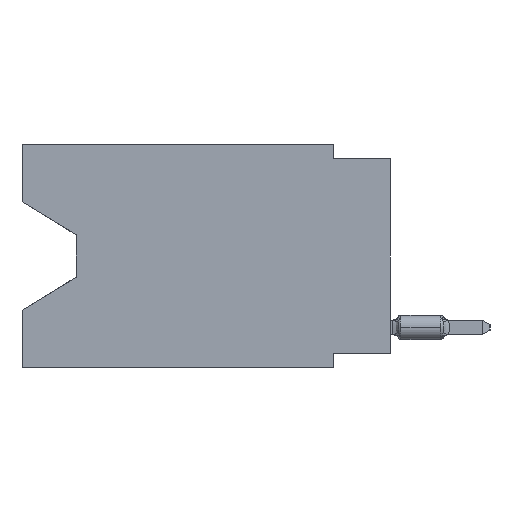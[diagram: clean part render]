
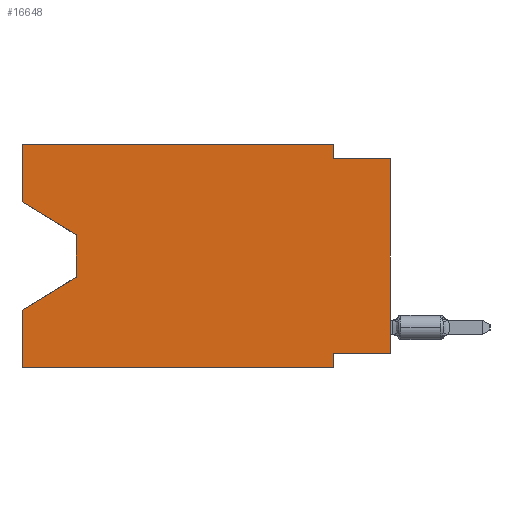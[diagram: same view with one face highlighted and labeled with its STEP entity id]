
A CAD part, left-side view. The second image highlights one B-rep face of the part: STEP entity #16648.
In plain terms, the highlighted planar face has unit normal (-1, 0, 0).
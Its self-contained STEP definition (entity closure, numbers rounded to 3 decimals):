
#16 = ORIENTED_EDGE ( 'NONE', *, *, #13307, .T. ) ;
#127 = EDGE_CURVE ( 'NONE', #4438, #49272, #79019, .T. ) ;
#498 = VERTEX_POINT ( 'NONE', #81264 ) ;
#1169 = CARTESIAN_POINT ( 'NONE',  ( 0., 0., 0. ) ) ;
#1260 = CARTESIAN_POINT ( 'NONE',  ( 0., 2.54, -0.635 ) ) ;
#3491 = ORIENTED_EDGE ( 'NONE', *, *, #4138, .F. ) ;
#4138 = EDGE_CURVE ( 'NONE', #498, #16381, #55338, .T. ) ;
#4438 = VERTEX_POINT ( 'NONE', #1260 ) ;
#4476 = DIRECTION ( 'NONE',  ( 0., 0., -1. ) ) ;
#4655 = AXIS2_PLACEMENT_3D ( 'NONE', #34418, #34010, #21267 ) ;
#6472 = ORIENTED_EDGE ( 'NONE', *, *, #15137, .T. ) ;
#6585 = CARTESIAN_POINT ( 'NONE',  ( 0., 13.97, -5.893 ) ) ;
#8643 = CARTESIAN_POINT ( 'NONE',  ( 0., 0., -9.271 ) ) ;
#10199 = VECTOR ( 'NONE', #22000, 1000. ) ;
#11069 = CARTESIAN_POINT ( 'NONE',  ( 0., 16.383, 0. ) ) ;
#11185 = ORIENTED_EDGE ( 'NONE', *, *, #53219, .T. ) ;
#11552 = VECTOR ( 'NONE', #78510, 1000. ) ;
#13207 = VECTOR ( 'NONE', #4476, 1000. ) ;
#13307 = EDGE_CURVE ( 'NONE', #77207, #38971, #28415, .T. ) ;
#13518 = VECTOR ( 'NONE', #74767, 1000. ) ;
#15030 = ORIENTED_EDGE ( 'NONE', *, *, #45302, .F. ) ;
#15137 = EDGE_CURVE ( 'NONE', #38971, #73579, #29148, .T. ) ;
#15429 = ORIENTED_EDGE ( 'NONE', *, *, #61055, .T. ) ;
#16334 = EDGE_CURVE ( 'NONE', #77207, #498, #55851, .T. ) ;
#16381 = VERTEX_POINT ( 'NONE', #30802 ) ;
#16648 = ADVANCED_FACE ( 'NONE', ( #27436 ), #47148, .F. ) ;
#16735 = CARTESIAN_POINT ( 'NONE',  ( 0., 16.383, -7.36 ) ) ;
#18494 = VECTOR ( 'NONE', #21832, 1000. ) ;
#19361 = LINE ( 'NONE', #68698, #32897 ) ;
#20143 = CARTESIAN_POINT ( 'NONE',  ( 0., 16.383, -9.906 ) ) ;
#21267 = DIRECTION ( 'NONE',  ( 0., 0., -1. ) ) ;
#21832 = DIRECTION ( 'NONE',  ( 0., -0.855, -0.519 ) ) ;
#22000 = DIRECTION ( 'NONE',  ( 0., 0., -1. ) ) ;
#22702 = DIRECTION ( 'NONE',  ( 0., -1., 0. ) ) ;
#23058 = VECTOR ( 'NONE', #34432, 1000. ) ;
#23804 = CARTESIAN_POINT ( 'NONE',  ( 0., 13.97, -4.013 ) ) ;
#27436 = FACE_OUTER_BOUND ( 'NONE', #63592, .T. ) ;
#28334 = CARTESIAN_POINT ( 'NONE',  ( 0., 16.383, -9.906 ) ) ;
#28415 = LINE ( 'NONE', #71963, #18494 ) ;
#29148 = LINE ( 'NONE', #23804, #13207 ) ;
#30026 = EDGE_CURVE ( 'NONE', #16381, #4438, #42361, .T. ) ;
#30802 = CARTESIAN_POINT ( 'NONE',  ( 0., 2.54, 0. ) ) ;
#32821 = VERTEX_POINT ( 'NONE', #16735 ) ;
#32897 = VECTOR ( 'NONE', #43634, 1000. ) ;
#33320 = LINE ( 'NONE', #8643, #11552 ) ;
#33664 = VECTOR ( 'NONE', #34979, 1000. ) ;
#34010 = DIRECTION ( 'NONE',  ( 1., 0., 0. ) ) ;
#34324 = ORIENTED_EDGE ( 'NONE', *, *, #80640, .F. ) ;
#34418 = CARTESIAN_POINT ( 'NONE',  ( 0., 16.383, 0. ) ) ;
#34432 = DIRECTION ( 'NONE',  ( 0., 0., 1. ) ) ;
#34979 = DIRECTION ( 'NONE',  ( 0., 0., -1. ) ) ;
#35494 = CARTESIAN_POINT ( 'NONE',  ( 0., 2.54, -9.271 ) ) ;
#36383 = VECTOR ( 'NONE', #57096, 1000. ) ;
#38610 = ORIENTED_EDGE ( 'NONE', *, *, #127, .F. ) ;
#38889 = EDGE_CURVE ( 'NONE', #64395, #80874, #51378, .T. ) ;
#38971 = VERTEX_POINT ( 'NONE', #72297 ) ;
#39202 = ORIENTED_EDGE ( 'NONE', *, *, #30026, .F. ) ;
#40088 = CARTESIAN_POINT ( 'NONE',  ( 0., 2.54, -9.906 ) ) ;
#41078 = ORIENTED_EDGE ( 'NONE', *, *, #16334, .F. ) ;
#42361 = LINE ( 'NONE', #66613, #33664 ) ;
#42679 = CARTESIAN_POINT ( 'NONE',  ( 0., 16.383, -2.546 ) ) ;
#43634 = DIRECTION ( 'NONE',  ( 0., 0., 1. ) ) ;
#44543 = CARTESIAN_POINT ( 'NONE',  ( 0., 16.383, 0. ) ) ;
#45220 = DIRECTION ( 'NONE',  ( 0., -1., 0. ) ) ;
#45302 = EDGE_CURVE ( 'NONE', #64395, #32821, #19361, .T. ) ;
#45835 = ORIENTED_EDGE ( 'NONE', *, *, #62761, .F. ) ;
#47148 = PLANE ( 'NONE',  #4655 ) ;
#48100 = VERTEX_POINT ( 'NONE', #35494 ) ;
#49272 = VERTEX_POINT ( 'NONE', #73292 ) ;
#50119 = CARTESIAN_POINT ( 'NONE',  ( 0., 0., -0.635 ) ) ;
#51378 = LINE ( 'NONE', #20143, #54349 ) ;
#52725 = VECTOR ( 'NONE', #80421, 1000. ) ;
#53219 = EDGE_CURVE ( 'NONE', #73579, #32821, #68644, .T. ) ;
#54349 = VECTOR ( 'NONE', #45220, 1000. ) ;
#55338 = LINE ( 'NONE', #44543, #52725 ) ;
#55851 = LINE ( 'NONE', #11069, #13518 ) ;
#56149 = CARTESIAN_POINT ( 'NONE',  ( 0., 13.97, -5.893 ) ) ;
#56397 = VERTEX_POINT ( 'NONE', #65940 ) ;
#57096 = DIRECTION ( 'NONE',  ( 0., 0.855, -0.519 ) ) ;
#61055 = EDGE_CURVE ( 'NONE', #56397, #49272, #63636, .T. ) ;
#62761 = EDGE_CURVE ( 'NONE', #48100, #80874, #65978, .T. ) ;
#63592 = EDGE_LOOP ( 'NONE', ( #16, #6472, #11185, #15030, #65575, #45835, #34324, #15429, #38610, #39202, #3491, #41078 ) ) ;
#63636 = LINE ( 'NONE', #1169, #23058 ) ;
#64395 = VERTEX_POINT ( 'NONE', #28334 ) ;
#65575 = ORIENTED_EDGE ( 'NONE', *, *, #38889, .T. ) ;
#65940 = CARTESIAN_POINT ( 'NONE',  ( 0., 0., -9.271 ) ) ;
#65978 = LINE ( 'NONE', #40088, #10199 ) ;
#66613 = CARTESIAN_POINT ( 'NONE',  ( 0., 2.54, 0. ) ) ;
#68020 = VECTOR ( 'NONE', #22702, 1000. ) ;
#68644 = LINE ( 'NONE', #6585, #36383 ) ;
#68698 = CARTESIAN_POINT ( 'NONE',  ( 0., 16.383, 0. ) ) ;
#71963 = CARTESIAN_POINT ( 'NONE',  ( 0., 16.383, -2.546 ) ) ;
#72297 = CARTESIAN_POINT ( 'NONE',  ( 0., 13.97, -4.013 ) ) ;
#73292 = CARTESIAN_POINT ( 'NONE',  ( 0., 0., -0.635 ) ) ;
#73579 = VERTEX_POINT ( 'NONE', #56149 ) ;
#74767 = DIRECTION ( 'NONE',  ( 0., 0., 1. ) ) ;
#77207 = VERTEX_POINT ( 'NONE', #42679 ) ;
#78033 = CARTESIAN_POINT ( 'NONE',  ( 0., 2.54, -9.906 ) ) ;
#78510 = DIRECTION ( 'NONE',  ( 0., 1., 0. ) ) ;
#79019 = LINE ( 'NONE', #50119, #68020 ) ;
#80421 = DIRECTION ( 'NONE',  ( 0., -1., 0. ) ) ;
#80640 = EDGE_CURVE ( 'NONE', #56397, #48100, #33320, .T. ) ;
#80874 = VERTEX_POINT ( 'NONE', #78033 ) ;
#81264 = CARTESIAN_POINT ( 'NONE',  ( 0., 16.383, 0. ) ) ;
